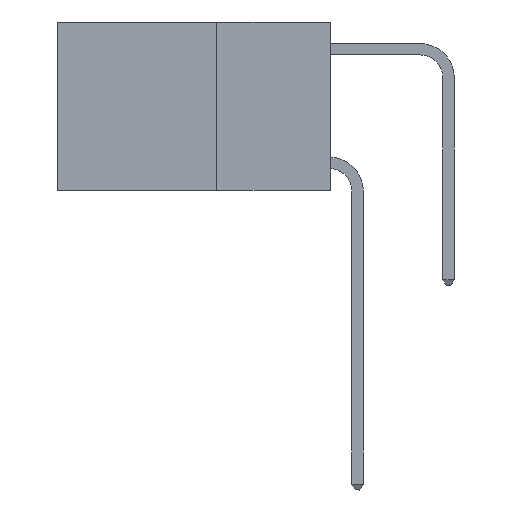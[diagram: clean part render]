
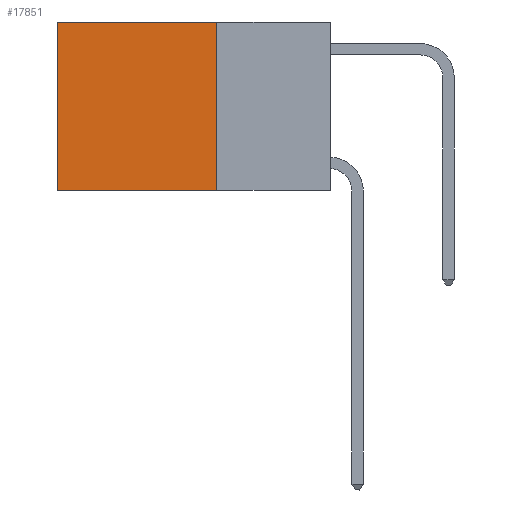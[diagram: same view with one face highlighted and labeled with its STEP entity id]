
A CAD part, left-side view. The second image highlights one B-rep face of the part: STEP entity #17851.
In plain terms, the highlighted planar face has unit normal (-1, 0, 0).
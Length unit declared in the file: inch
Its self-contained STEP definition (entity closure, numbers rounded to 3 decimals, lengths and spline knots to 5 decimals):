
#70 = CARTESIAN_POINT ( 'NONE',  ( 0.2625, 0.6, 0. ) ) ;
#150 = VECTOR ( 'NONE', #15252, 39.37008 ) ;
#178 = CARTESIAN_POINT ( 'NONE',  ( 0.2625, 0.25, 0. ) ) ;
#438 = VERTEX_POINT ( 'NONE', #4899 ) ;
#1445 = ORIENTED_EDGE ( 'NONE', *, *, #7079, .T. ) ;
#2374 = LINE ( 'NONE', #17390, #10771 ) ;
#2972 = VERTEX_POINT ( 'NONE', #9605 ) ;
#3181 = LINE ( 'NONE', #6329, #11598 ) ;
#4899 = CARTESIAN_POINT ( 'NONE',  ( 0.2625, 0.25, 0. ) ) ;
#5227 = VERTEX_POINT ( 'NONE', #14365 ) ;
#5763 = CARTESIAN_POINT ( 'NONE',  ( 0.2625, 0.6, 0. ) ) ;
#6329 = CARTESIAN_POINT ( 'NONE',  ( 0.2625, 0.25, -0.37 ) ) ;
#7079 = EDGE_CURVE ( 'NONE', #14650, #2972, #7909, .T. ) ;
#7909 = LINE ( 'NONE', #5763, #16195 ) ;
#8395 = DIRECTION ( 'NONE',  ( 1., 0., 0. ) ) ;
#9115 = LINE ( 'NONE', #178, #150 ) ;
#9590 = ORIENTED_EDGE ( 'NONE', *, *, #19008, .T. ) ;
#9605 = CARTESIAN_POINT ( 'NONE',  ( 0.2625, 0.6, -0.37 ) ) ;
#10771 = VECTOR ( 'NONE', #19026, 39.37008 ) ;
#11005 = EDGE_CURVE ( 'NONE', #438, #5227, #9115, .T. ) ;
#11412 = ORIENTED_EDGE ( 'NONE', *, *, #11005, .F. ) ;
#11598 = VECTOR ( 'NONE', #17892, 39.37008 ) ;
#11626 = FACE_OUTER_BOUND ( 'NONE', #17778, .T. ) ;
#14365 = CARTESIAN_POINT ( 'NONE',  ( 0.2625, 0.25, -0.37 ) ) ;
#14650 = VERTEX_POINT ( 'NONE', #70 ) ;
#14788 = ORIENTED_EDGE ( 'NONE', *, *, #15084, .F. ) ;
#14993 = CARTESIAN_POINT ( 'NONE',  ( 0.2625, 0.25, 0. ) ) ;
#15084 = EDGE_CURVE ( 'NONE', #5227, #2972, #3181, .T. ) ;
#15252 = DIRECTION ( 'NONE',  ( 0., 0., -1. ) ) ;
#16195 = VECTOR ( 'NONE', #18987, 39.37008 ) ;
#16963 = AXIS2_PLACEMENT_3D ( 'NONE', #14993, #8395, #19882 ) ;
#17390 = CARTESIAN_POINT ( 'NONE',  ( 0.2625, 0.25, 0. ) ) ;
#17778 = EDGE_LOOP ( 'NONE', ( #1445, #14788, #11412, #9590 ) ) ;
#17851 = ADVANCED_FACE ( 'NONE', ( #11626 ), #21430, .F. ) ;
#17892 = DIRECTION ( 'NONE',  ( 0., 1., 0. ) ) ;
#18987 = DIRECTION ( 'NONE',  ( 0., 0., -1. ) ) ;
#19008 = EDGE_CURVE ( 'NONE', #438, #14650, #2374, .T. ) ;
#19026 = DIRECTION ( 'NONE',  ( 0., 1., 0. ) ) ;
#19882 = DIRECTION ( 'NONE',  ( 0., 0., -1. ) ) ;
#21430 = PLANE ( 'NONE',  #16963 ) ;
